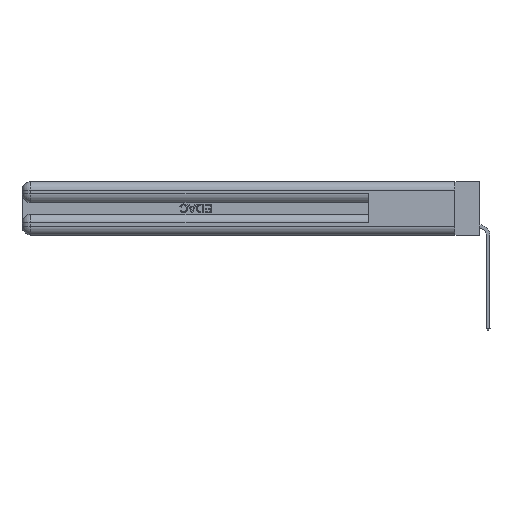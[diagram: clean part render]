
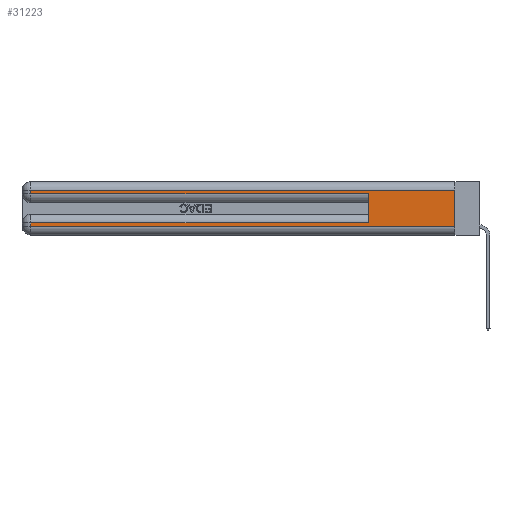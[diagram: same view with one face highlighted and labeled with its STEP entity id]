
A CAD part, left-side view. The second image highlights one B-rep face of the part: STEP entity #31223.
In plain terms, the highlighted planar face has unit normal (-1, 0, 0).
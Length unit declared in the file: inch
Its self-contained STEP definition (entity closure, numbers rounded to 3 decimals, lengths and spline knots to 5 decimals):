
#44 = CARTESIAN_POINT ( 'NONE',  ( 0., 2.94, 0.37 ) ) ;
#174 = VECTOR ( 'NONE', #7608, 39.37008 ) ;
#584 = CARTESIAN_POINT ( 'NONE',  ( 0., 2.94, 0.285 ) ) ;
#1173 = CARTESIAN_POINT ( 'NONE',  ( 0., 0.6, 0.285 ) ) ;
#1736 = EDGE_CURVE ( 'NONE', #10048, #28496, #3729, .T. ) ;
#2627 = CARTESIAN_POINT ( 'NONE',  ( 0., 0., 0.31 ) ) ;
#3729 = LINE ( 'NONE', #8268, #16222 ) ;
#4037 = CARTESIAN_POINT ( 'NONE',  ( 0., 0., 0.31 ) ) ;
#4448 = EDGE_CURVE ( 'NONE', #6984, #28496, #24773, .T. ) ;
#4461 = DIRECTION ( 'NONE',  ( 0., -1., 0. ) ) ;
#6545 = VECTOR ( 'NONE', #10068, 39.37008 ) ;
#6571 = VERTEX_POINT ( 'NONE', #4037 ) ;
#6984 = VERTEX_POINT ( 'NONE', #584 ) ;
#7608 = DIRECTION ( 'NONE',  ( 0., 0., -1. ) ) ;
#7776 = ORIENTED_EDGE ( 'NONE', *, *, #1736, .F. ) ;
#8068 = CARTESIAN_POINT ( 'NONE',  ( 0., 0., 0.06 ) ) ;
#8268 = CARTESIAN_POINT ( 'NONE',  ( 0., 0.6, 0.145 ) ) ;
#8597 = LINE ( 'NONE', #8963, #30397 ) ;
#8937 = ORIENTED_EDGE ( 'NONE', *, *, #16487, .T. ) ;
#8963 = CARTESIAN_POINT ( 'NONE',  ( 0., 0., 0.06 ) ) ;
#9814 = DIRECTION ( 'NONE',  ( 0., 0., -1. ) ) ;
#10048 = VERTEX_POINT ( 'NONE', #20067 ) ;
#10068 = DIRECTION ( 'NONE',  ( 0., 1., 0. ) ) ;
#10212 = LINE ( 'NONE', #44, #15230 ) ;
#10223 = DIRECTION ( 'NONE',  ( 0., 1., 0. ) ) ;
#10548 = EDGE_CURVE ( 'NONE', #14135, #6984, #10212, .T. ) ;
#10611 = DIRECTION ( 'NONE',  ( 0., 0., -1. ) ) ;
#10680 = CARTESIAN_POINT ( 'NONE',  ( 0., 2.94, 0.06 ) ) ;
#10717 = CARTESIAN_POINT ( 'NONE',  ( 0., 2.94, 0.31 ) ) ;
#11305 = AXIS2_PLACEMENT_3D ( 'NONE', #20367, #25219, #10611 ) ;
#11477 = DIRECTION ( 'NONE',  ( 0., -1., 0. ) ) ;
#12329 = CARTESIAN_POINT ( 'NONE',  ( 0., 0., 0.37 ) ) ;
#13003 = LINE ( 'NONE', #2627, #25161 ) ;
#13174 = VERTEX_POINT ( 'NONE', #8068 ) ;
#14135 = VERTEX_POINT ( 'NONE', #10717 ) ;
#14722 = VECTOR ( 'NONE', #9814, 39.37008 ) ;
#14765 = ORIENTED_EDGE ( 'NONE', *, *, #22359, .F. ) ;
#15072 = DIRECTION ( 'NONE',  ( 0., 0., -1. ) ) ;
#15113 = FACE_OUTER_BOUND ( 'NONE', #22308, .T. ) ;
#15230 = VECTOR ( 'NONE', #15072, 39.37008 ) ;
#16222 = VECTOR ( 'NONE', #27857, 39.37008 ) ;
#16487 = EDGE_CURVE ( 'NONE', #6571, #14135, #13003, .T. ) ;
#17468 = CARTESIAN_POINT ( 'NONE',  ( 0., 2.94, 0.37 ) ) ;
#17908 = VERTEX_POINT ( 'NONE', #10680 ) ;
#20042 = LINE ( 'NONE', #17468, #174 ) ;
#20067 = CARTESIAN_POINT ( 'NONE',  ( 0., 0.6, 0.085 ) ) ;
#20367 = CARTESIAN_POINT ( 'NONE',  ( 0., 0., 0.37 ) ) ;
#20518 = ORIENTED_EDGE ( 'NONE', *, *, #29110, .T. ) ;
#22308 = EDGE_LOOP ( 'NONE', ( #14765, #8937, #22764, #23540, #7776, #30360, #25429, #20518 ) ) ;
#22359 = EDGE_CURVE ( 'NONE', #6571, #13174, #27647, .T. ) ;
#22764 = ORIENTED_EDGE ( 'NONE', *, *, #10548, .T. ) ;
#22791 = PLANE ( 'NONE',  #11305 ) ;
#23540 = ORIENTED_EDGE ( 'NONE', *, *, #4448, .T. ) ;
#24033 = VECTOR ( 'NONE', #4461, 39.37008 ) ;
#24773 = LINE ( 'NONE', #28957, #24033 ) ;
#25161 = VECTOR ( 'NONE', #10223, 39.37008 ) ;
#25219 = DIRECTION ( 'NONE',  ( 1., 0., 0. ) ) ;
#25376 = LINE ( 'NONE', #27155, #6545 ) ;
#25429 = ORIENTED_EDGE ( 'NONE', *, *, #31732, .T. ) ;
#27155 = CARTESIAN_POINT ( 'NONE',  ( 0., 0., 0.085 ) ) ;
#27647 = LINE ( 'NONE', #12329, #14722 ) ;
#27857 = DIRECTION ( 'NONE',  ( 0., 0., 1. ) ) ;
#28496 = VERTEX_POINT ( 'NONE', #1173 ) ;
#28957 = CARTESIAN_POINT ( 'NONE',  ( 0., 0., 0.285 ) ) ;
#29110 = EDGE_CURVE ( 'NONE', #17908, #13174, #8597, .T. ) ;
#30242 = CARTESIAN_POINT ( 'NONE',  ( 0., 2.94, 0.085 ) ) ;
#30360 = ORIENTED_EDGE ( 'NONE', *, *, #31073, .T. ) ;
#30397 = VECTOR ( 'NONE', #11477, 39.37008 ) ;
#30663 = VERTEX_POINT ( 'NONE', #30242 ) ;
#31073 = EDGE_CURVE ( 'NONE', #10048, #30663, #25376, .T. ) ;
#31223 = ADVANCED_FACE ( 'NONE', ( #15113 ), #22791, .F. ) ;
#31732 = EDGE_CURVE ( 'NONE', #30663, #17908, #20042, .T. ) ;
